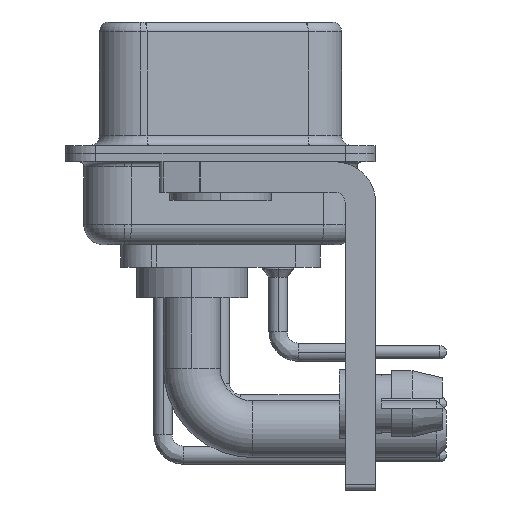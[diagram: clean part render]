
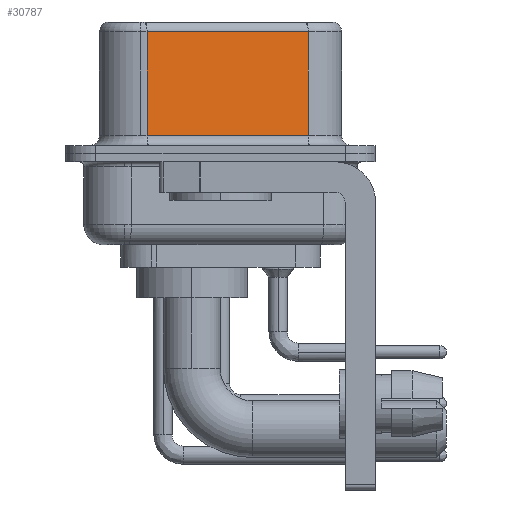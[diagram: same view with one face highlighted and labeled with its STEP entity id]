
A CAD part, left-side view. The second image highlights one B-rep face of the part: STEP entity #30787.
In plain terms, the highlighted planar face has unit normal (-0.985, -0.174, 0).
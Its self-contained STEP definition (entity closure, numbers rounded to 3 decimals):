
#2027 = CARTESIAN_POINT ( 'NONE',  ( 3.73, 3.628, 6.52 ) ) ;
#2212 = LINE ( 'NONE', #2027, #35705 ) ;
#2286 = DIRECTION ( 'NONE',  ( -0.174, 0.985, 0. ) ) ;
#2587 = VECTOR ( 'NONE', #34842, 1000. ) ;
#2731 = VERTEX_POINT ( 'NONE', #24042 ) ;
#3382 = VECTOR ( 'NONE', #15136, 1000. ) ;
#4772 = ORIENTED_EDGE ( 'NONE', *, *, #17268, .T. ) ;
#5732 = CARTESIAN_POINT ( 'NONE',  ( 5.132, -4.322, 6.52 ) ) ;
#5792 = CARTESIAN_POINT ( 'NONE',  ( 3.73, 3.628, 6.02 ) ) ;
#7288 = EDGE_CURVE ( 'NONE', #2731, #18329, #11517, .T. ) ;
#9969 = CARTESIAN_POINT ( 'NONE',  ( 5.132, -4.322, 6.02 ) ) ;
#10034 = CARTESIAN_POINT ( 'NONE',  ( 5.132, -4.322, 6.02 ) ) ;
#10144 = EDGE_CURVE ( 'NONE', #18348, #18329, #31816, .T. ) ;
#10313 = EDGE_CURVE ( 'NONE', #18348, #20685, #20706, .T. ) ;
#11281 = DIRECTION ( 'NONE',  ( 0., 0., -1. ) ) ;
#11316 = EDGE_LOOP ( 'NONE', ( #30090, #25842, #4772, #18311 ) ) ;
#11517 = LINE ( 'NONE', #31684, #2587 ) ;
#15136 = DIRECTION ( 'NONE',  ( -0.174, 0.985, 0. ) ) ;
#15949 = AXIS2_PLACEMENT_3D ( 'NONE', #33774, #19320, #2286 ) ;
#17268 = EDGE_CURVE ( 'NONE', #20685, #2731, #2212, .T. ) ;
#18311 = ORIENTED_EDGE ( 'NONE', *, *, #7288, .T. ) ;
#18329 = VERTEX_POINT ( 'NONE', #23731 ) ;
#18348 = VERTEX_POINT ( 'NONE', #10034 ) ;
#18960 = FACE_OUTER_BOUND ( 'NONE', #11316, .T. ) ;
#19320 = DIRECTION ( 'NONE',  ( 0.985, 0.174, 0. ) ) ;
#19923 = VECTOR ( 'NONE', #11281, 1000. ) ;
#20685 = VERTEX_POINT ( 'NONE', #5792 ) ;
#20706 = LINE ( 'NONE', #9969, #3382 ) ;
#23731 = CARTESIAN_POINT ( 'NONE',  ( 5.132, -4.322, 0.9 ) ) ;
#24042 = CARTESIAN_POINT ( 'NONE',  ( 3.73, 3.628, 0.9 ) ) ;
#25842 = ORIENTED_EDGE ( 'NONE', *, *, #10313, .T. ) ;
#27757 = DIRECTION ( 'NONE',  ( 0., 0., -1. ) ) ;
#30090 = ORIENTED_EDGE ( 'NONE', *, *, #10144, .F. ) ;
#30787 = ADVANCED_FACE ( 'NONE', ( #18960 ), #32488, .F. ) ;
#31684 = CARTESIAN_POINT ( 'NONE',  ( 5.132, -4.322, 0.9 ) ) ;
#31816 = LINE ( 'NONE', #5732, #19923 ) ;
#32488 = PLANE ( 'NONE',  #15949 ) ;
#33774 = CARTESIAN_POINT ( 'NONE',  ( 5.132, -4.322, 6.52 ) ) ;
#34842 = DIRECTION ( 'NONE',  ( 0.174, -0.985, 0. ) ) ;
#35705 = VECTOR ( 'NONE', #27757, 1000. ) ;
